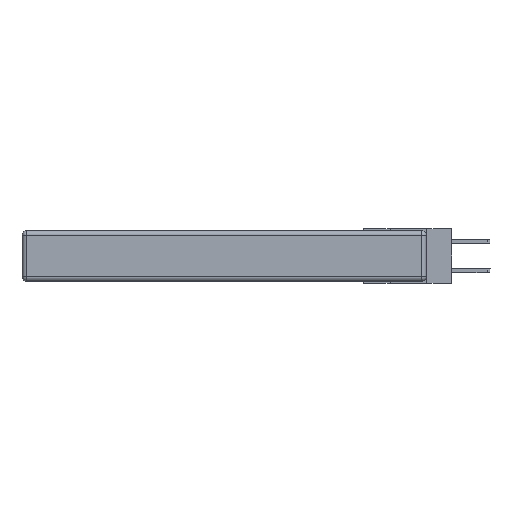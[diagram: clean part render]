
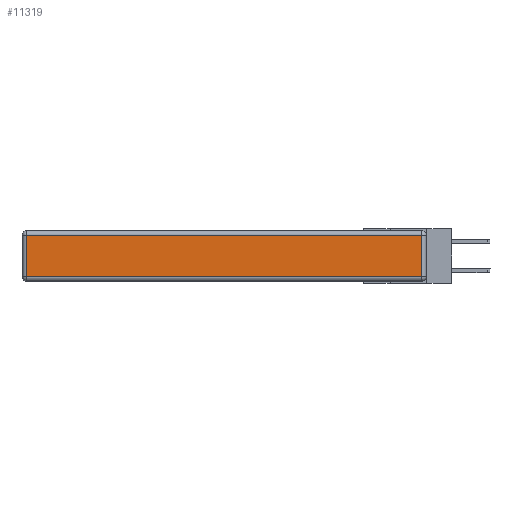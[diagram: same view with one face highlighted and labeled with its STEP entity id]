
A CAD part, left-side view. The second image highlights one B-rep face of the part: STEP entity #11319.
In plain terms, the highlighted planar face has unit normal (-1, 0, 0).
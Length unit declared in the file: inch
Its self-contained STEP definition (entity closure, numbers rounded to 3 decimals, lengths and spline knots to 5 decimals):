
#636 = DIRECTION ( 'NONE',  ( -1., 0., 0. ) ) ;
#783 = EDGE_CURVE ( 'NONE', #10639, #6671, #5376, .T. ) ;
#1051 = VECTOR ( 'NONE', #3516, 39.37008 ) ;
#1392 = DIRECTION ( 'NONE',  ( 0., -1., 0. ) ) ;
#1944 = ORIENTED_EDGE ( 'NONE', *, *, #11144, .T. ) ;
#2104 = EDGE_CURVE ( 'NONE', #6684, #6861, #9477, .T. ) ;
#2301 = CARTESIAN_POINT ( 'NONE',  ( 0., 0.03, -0.343 ) ) ;
#3516 = DIRECTION ( 'NONE',  ( 0., 1., 0. ) ) ;
#3827 = VECTOR ( 'NONE', #1392, 39.37008 ) ;
#4029 = CARTESIAN_POINT ( 'NONE',  ( 0., 2.72, -0.03 ) ) ;
#4615 = ORIENTED_EDGE ( 'NONE', *, *, #783, .T. ) ;
#4710 = LINE ( 'NONE', #6088, #3827 ) ;
#4846 = FACE_OUTER_BOUND ( 'NONE', #6844, .T. ) ;
#5121 = CARTESIAN_POINT ( 'NONE',  ( 0., 2.72, -0.313 ) ) ;
#5318 = CARTESIAN_POINT ( 'NONE',  ( 0., 0., -0.343 ) ) ;
#5354 = CARTESIAN_POINT ( 'NONE',  ( 0., 2.75, -0.03 ) ) ;
#5376 = LINE ( 'NONE', #2301, #8152 ) ;
#5836 = CARTESIAN_POINT ( 'NONE',  ( 0., 2.72, -0.343 ) ) ;
#6088 = CARTESIAN_POINT ( 'NONE',  ( 0., 0., -0.313 ) ) ;
#6671 = VERTEX_POINT ( 'NONE', #6864 ) ;
#6684 = VERTEX_POINT ( 'NONE', #4029 ) ;
#6844 = EDGE_LOOP ( 'NONE', ( #1944, #4615, #10435, #8029 ) ) ;
#6861 = VERTEX_POINT ( 'NONE', #5121 ) ;
#6864 = CARTESIAN_POINT ( 'NONE',  ( 0., 0.03, -0.03 ) ) ;
#7181 = DIRECTION ( 'NONE',  ( 0., 0., 1. ) ) ;
#7195 = DIRECTION ( 'NONE',  ( 0., 0., 1. ) ) ;
#7624 = LINE ( 'NONE', #5354, #1051 ) ;
#8029 = ORIENTED_EDGE ( 'NONE', *, *, #2104, .T. ) ;
#8152 = VECTOR ( 'NONE', #7181, 39.37008 ) ;
#8488 = AXIS2_PLACEMENT_3D ( 'NONE', #5318, #636, #7195 ) ;
#9092 = PLANE ( 'NONE',  #8488 ) ;
#9477 = LINE ( 'NONE', #5836, #9924 ) ;
#9924 = VECTOR ( 'NONE', #11506, 39.37008 ) ;
#10435 = ORIENTED_EDGE ( 'NONE', *, *, #11318, .T. ) ;
#10639 = VERTEX_POINT ( 'NONE', #11045 ) ;
#11045 = CARTESIAN_POINT ( 'NONE',  ( 0., 0.03, -0.313 ) ) ;
#11144 = EDGE_CURVE ( 'NONE', #6861, #10639, #4710, .T. ) ;
#11318 = EDGE_CURVE ( 'NONE', #6671, #6684, #7624, .T. ) ;
#11319 = ADVANCED_FACE ( 'NONE', ( #4846 ), #9092, .T. ) ;
#11506 = DIRECTION ( 'NONE',  ( 0., 0., -1. ) ) ;
